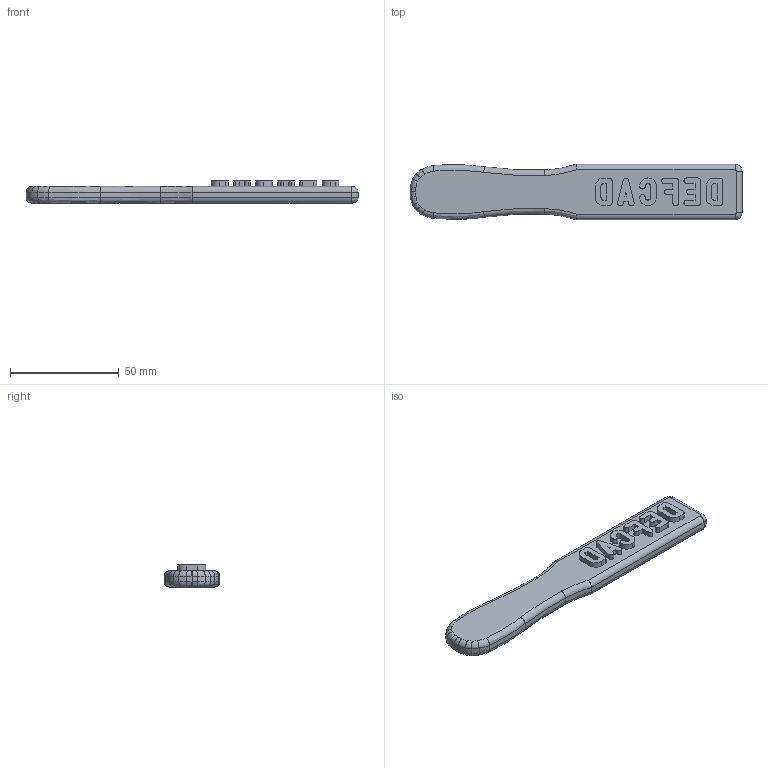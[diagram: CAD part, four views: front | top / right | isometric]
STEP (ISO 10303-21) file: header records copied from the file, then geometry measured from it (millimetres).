
FILE_DESCRIPTION(('Open CASCADE Model'),'2;1');
FILE_NAME('Open CASCADE Shape Model','2013-05-28T05:07:35',('Author'),( 'Open CASCADE'),'Open CASCADE STEP processor 6.1','Open CASCADE 6.1' ,'Unknown');
FILE_SCHEMA(('AUTOMOTIVE_DESIGN_CC2 { 1 2 10303 214 -1 1 5 4 }'));
Length unit declared in the file: millimetre
Products named in the file (3): Product 1; Product 1.1; Product 1.2
Assembly tree (2 placements, depth 2):
  Product 1
    Product 1.1
    Product 1.2
Bounding box: 152.4 x 25.4 x 10.16 mm (x, y, z)
Volume: 27306.6 mm3; surface area: 10105.1 mm2
Topology: 1 solids, 3 shells, 197 faces, 508 edges, 298 vertices
Faces by surface type: bspline 176, plane 21
Entity records: 15785 total; most frequent: CARTESIAN_POINT 8743, ORIENTED_EDGE 936, PCURVE 936, DEFINITIONAL_REPRESENTATION 936, DIRECTION 669, LINE 639, VECTOR 639, EDGE_CURVE 472
